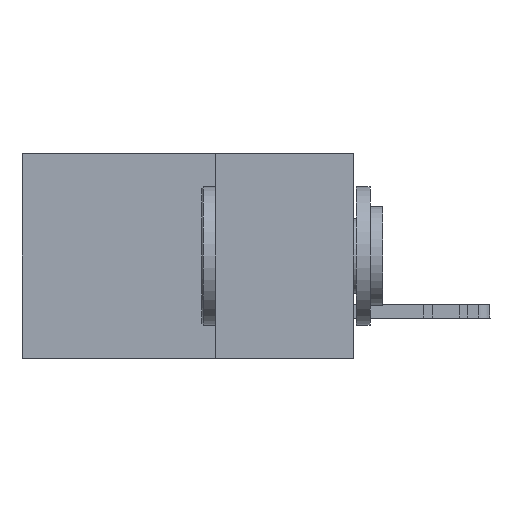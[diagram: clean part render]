
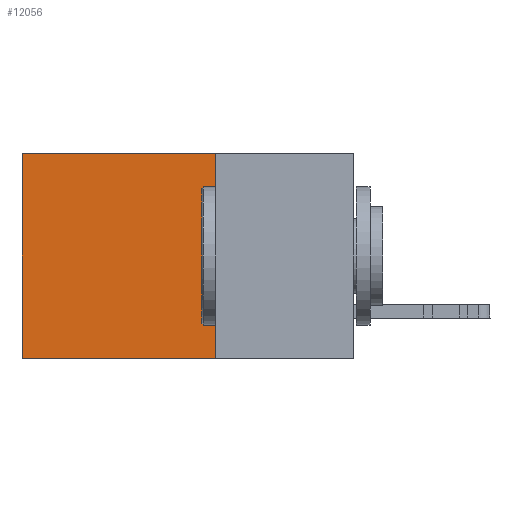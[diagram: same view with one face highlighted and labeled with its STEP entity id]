
A CAD part, left-side view. The second image highlights one B-rep face of the part: STEP entity #12056.
In plain terms, the highlighted planar face has unit normal (-1, 0, 0).
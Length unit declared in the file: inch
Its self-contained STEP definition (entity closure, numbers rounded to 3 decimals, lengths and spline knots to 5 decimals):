
#1372 = DIRECTION ( 'NONE',  ( 0., 1., 0. ) ) ;
#2522 = VECTOR ( 'NONE', #1372, 39.37008 ) ;
#3114 = CARTESIAN_POINT ( 'NONE',  ( 0.2875, 0.6, 0. ) ) ;
#3366 = PLANE ( 'NONE',  #21209 ) ;
#3491 = EDGE_CURVE ( 'NONE', #39232, #41036, #17309, .T. ) ;
#4800 = EDGE_LOOP ( 'NONE', ( #25613, #43190, #22372, #38432 ) ) ;
#6524 = VECTOR ( 'NONE', #29551, 39.37008 ) ;
#8732 = CARTESIAN_POINT ( 'NONE',  ( 0.2875, 0.6, 0. ) ) ;
#9429 = VECTOR ( 'NONE', #35951, 39.37008 ) ;
#9482 = LINE ( 'NONE', #35768, #9429 ) ;
#12056 = ADVANCED_FACE ( 'NONE', ( #23683 ), #3366, .F. ) ;
#12152 = DIRECTION ( 'NONE',  ( 0., 0., -1. ) ) ;
#14404 = LINE ( 'NONE', #3114, #32286 ) ;
#15580 = EDGE_CURVE ( 'NONE', #27389, #41036, #14404, .T. ) ;
#17309 = LINE ( 'NONE', #37048, #6524 ) ;
#19846 = DIRECTION ( 'NONE',  ( 1., 0., 0. ) ) ;
#20499 = CARTESIAN_POINT ( 'NONE',  ( 0.2875, 0.25, 0. ) ) ;
#21042 = EDGE_CURVE ( 'NONE', #32915, #27389, #24620, .T. ) ;
#21209 = AXIS2_PLACEMENT_3D ( 'NONE', #26165, #19846, #12152 ) ;
#22372 = ORIENTED_EDGE ( 'NONE', *, *, #44914, .F. ) ;
#23683 = FACE_OUTER_BOUND ( 'NONE', #4800, .T. ) ;
#24620 = LINE ( 'NONE', #20499, #2522 ) ;
#25613 = ORIENTED_EDGE ( 'NONE', *, *, #15580, .T. ) ;
#26165 = CARTESIAN_POINT ( 'NONE',  ( 0.2875, 0.25, 0. ) ) ;
#26599 = CARTESIAN_POINT ( 'NONE',  ( 0.2875, 0.6, -0.37 ) ) ;
#27389 = VERTEX_POINT ( 'NONE', #8732 ) ;
#29551 = DIRECTION ( 'NONE',  ( 0., 1., 0. ) ) ;
#32286 = VECTOR ( 'NONE', #44716, 39.37008 ) ;
#32915 = VERTEX_POINT ( 'NONE', #48149 ) ;
#35768 = CARTESIAN_POINT ( 'NONE',  ( 0.2875, 0.25, 0. ) ) ;
#35951 = DIRECTION ( 'NONE',  ( 0., 0., -1. ) ) ;
#37048 = CARTESIAN_POINT ( 'NONE',  ( 0.2875, 0.25, -0.37 ) ) ;
#38432 = ORIENTED_EDGE ( 'NONE', *, *, #21042, .T. ) ;
#39232 = VERTEX_POINT ( 'NONE', #45038 ) ;
#41036 = VERTEX_POINT ( 'NONE', #26599 ) ;
#43190 = ORIENTED_EDGE ( 'NONE', *, *, #3491, .F. ) ;
#44716 = DIRECTION ( 'NONE',  ( 0., 0., -1. ) ) ;
#44914 = EDGE_CURVE ( 'NONE', #32915, #39232, #9482, .T. ) ;
#45038 = CARTESIAN_POINT ( 'NONE',  ( 0.2875, 0.25, -0.37 ) ) ;
#48149 = CARTESIAN_POINT ( 'NONE',  ( 0.2875, 0.25, 0. ) ) ;
